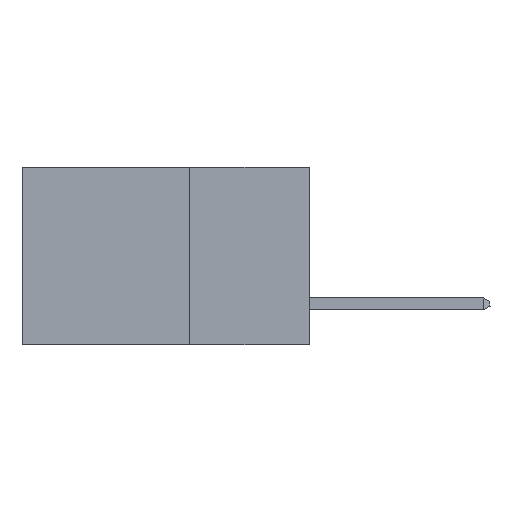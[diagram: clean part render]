
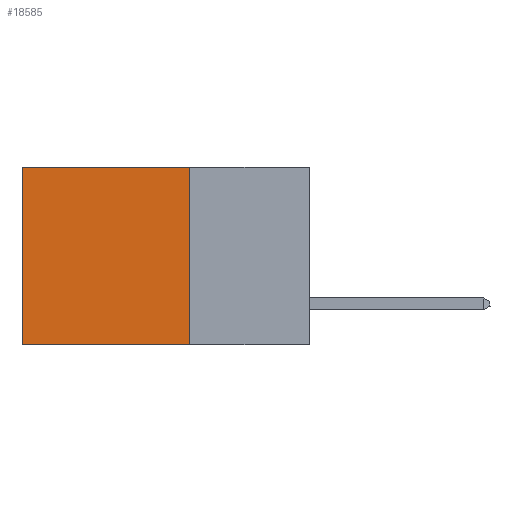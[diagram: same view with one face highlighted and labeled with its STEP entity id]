
A CAD part, left-side view. The second image highlights one B-rep face of the part: STEP entity #18585.
In plain terms, the highlighted planar face has unit normal (-1, 0, 0).
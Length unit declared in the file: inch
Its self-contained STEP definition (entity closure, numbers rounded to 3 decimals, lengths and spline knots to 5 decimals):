
#415 = LINE ( 'NONE', #28630, #35381 ) ;
#1529 = DIRECTION ( 'NONE',  ( 0., 0., -1. ) ) ;
#2022 = CARTESIAN_POINT ( 'NONE',  ( 0.2875, 0.25, 0. ) ) ;
#4046 = EDGE_CURVE ( 'NONE', #5885, #15878, #415, .T. ) ;
#4712 = VECTOR ( 'NONE', #19138, 39.37008 ) ;
#5885 = VERTEX_POINT ( 'NONE', #26430 ) ;
#6013 = VECTOR ( 'NONE', #17004, 39.37008 ) ;
#7237 = PLANE ( 'NONE',  #18609 ) ;
#9060 = ORIENTED_EDGE ( 'NONE', *, *, #41187, .F. ) ;
#9878 = CARTESIAN_POINT ( 'NONE',  ( 0.2875, 0.6, -0.37 ) ) ;
#10803 = CARTESIAN_POINT ( 'NONE',  ( 0.2875, 0.25, 0. ) ) ;
#14647 = VECTOR ( 'NONE', #31046, 39.37008 ) ;
#15188 = FACE_OUTER_BOUND ( 'NONE', #27727, .T. ) ;
#15653 = VERTEX_POINT ( 'NONE', #39008 ) ;
#15878 = VERTEX_POINT ( 'NONE', #9878 ) ;
#17004 = DIRECTION ( 'NONE',  ( 0., 1., 0. ) ) ;
#18585 = ADVANCED_FACE ( 'NONE', ( #15188 ), #7237, .F. ) ;
#18609 = AXIS2_PLACEMENT_3D ( 'NONE', #10803, #24442, #34522 ) ;
#19138 = DIRECTION ( 'NONE',  ( 0., 0., -1. ) ) ;
#20503 = ORIENTED_EDGE ( 'NONE', *, *, #42602, .F. ) ;
#23295 = LINE ( 'NONE', #23757, #4712 ) ;
#23757 = CARTESIAN_POINT ( 'NONE',  ( 0.2875, 0.25, 0. ) ) ;
#24442 = DIRECTION ( 'NONE',  ( 1., 0., 0. ) ) ;
#25131 = LINE ( 'NONE', #34223, #6013 ) ;
#26082 = VERTEX_POINT ( 'NONE', #2022 ) ;
#26430 = CARTESIAN_POINT ( 'NONE',  ( 0.2875, 0.6, 0. ) ) ;
#26864 = LINE ( 'NONE', #34768, #14647 ) ;
#27727 = EDGE_LOOP ( 'NONE', ( #32929, #20503, #9060, #30198 ) ) ;
#28630 = CARTESIAN_POINT ( 'NONE',  ( 0.2875, 0.6, 0. ) ) ;
#30198 = ORIENTED_EDGE ( 'NONE', *, *, #43904, .T. ) ;
#31046 = DIRECTION ( 'NONE',  ( 0., 1., 0. ) ) ;
#32929 = ORIENTED_EDGE ( 'NONE', *, *, #4046, .T. ) ;
#34223 = CARTESIAN_POINT ( 'NONE',  ( 0.2875, 0.25, 0. ) ) ;
#34522 = DIRECTION ( 'NONE',  ( 0., 0., -1. ) ) ;
#34768 = CARTESIAN_POINT ( 'NONE',  ( 0.2875, 0.25, -0.37 ) ) ;
#35381 = VECTOR ( 'NONE', #1529, 39.37008 ) ;
#39008 = CARTESIAN_POINT ( 'NONE',  ( 0.2875, 0.25, -0.37 ) ) ;
#41187 = EDGE_CURVE ( 'NONE', #26082, #15653, #23295, .T. ) ;
#42602 = EDGE_CURVE ( 'NONE', #15653, #15878, #26864, .T. ) ;
#43904 = EDGE_CURVE ( 'NONE', #26082, #5885, #25131, .T. ) ;
